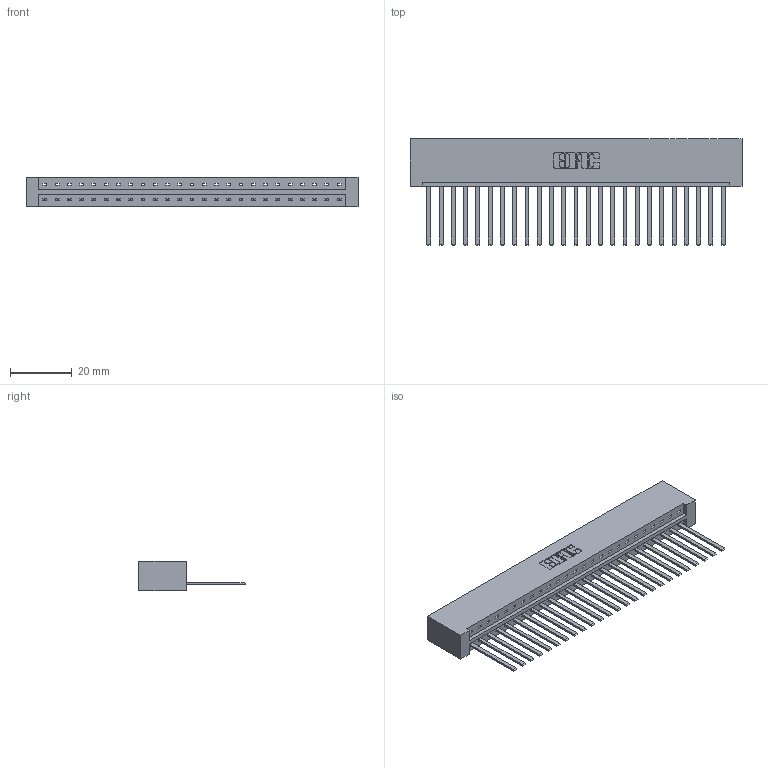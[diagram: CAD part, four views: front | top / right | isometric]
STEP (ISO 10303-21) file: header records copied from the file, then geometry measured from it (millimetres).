
FILE_DESCRIPTION (( 'STEP AP203' ), '1' );
FILE_NAME ('333-025-544-101.STEP', '2018-08-02T12:13:40', ( '' ), ( '' ), 'SwSTEP 2.0', 'SolidWorks 2016', '' );
FILE_SCHEMA (( 'CONFIG_CONTROL_DESIGN' ));
Length unit declared in the file: inch
Products named in the file (3): 333 Part_Lugless; 345-292-001_345-293-144; 333-025-544-101
Assembly tree (26 placements, depth 2):
  333-025-544-101
    333 Part_Lugless
    345-292-001_345-293-144  x25
Bounding box: 107.31 x 34.3 x 9.4 mm (x, y, z)
Volume: 11555 mm3; surface area: 13289 mm2
Topology: 26 solids, 26 shells, 1406 faces, 4237 edges, 2790 vertices
Faces by surface type: plane 1016, cylinder 390
Entity records: 17021 total; most frequent: CARTESIAN_POINT 2945, ORIENTED_EDGE 2906, DIRECTION 2507, EDGE_CURVE 1453, LINE 1337, VECTOR 1337, VERTEX_POINT 966, AXIS2_PLACEMENT_3D 585
